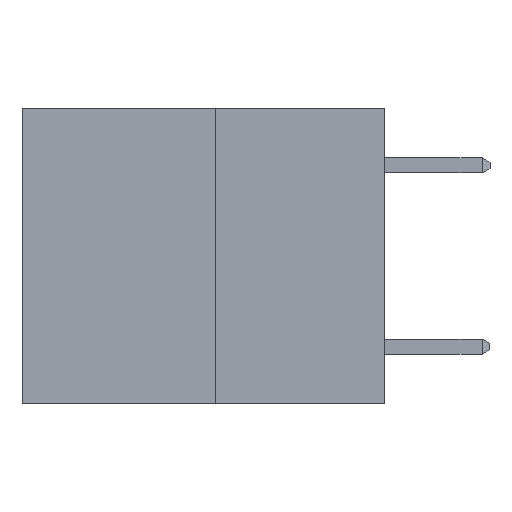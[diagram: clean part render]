
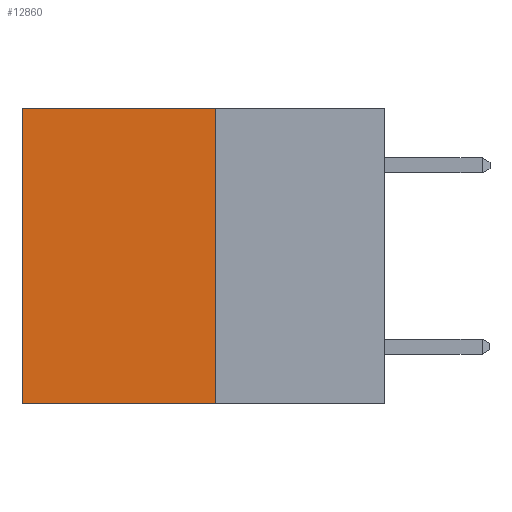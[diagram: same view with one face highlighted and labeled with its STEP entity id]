
A CAD part, left-side view. The second image highlights one B-rep face of the part: STEP entity #12860.
In plain terms, the highlighted planar face has unit normal (-1, 0, 0).
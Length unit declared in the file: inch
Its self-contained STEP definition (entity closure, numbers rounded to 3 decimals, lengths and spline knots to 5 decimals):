
#2913 = VECTOR ( 'NONE', #9610, 39.37008 ) ;
#2992 = DIRECTION ( 'NONE',  ( 1., 0., 0. ) ) ;
#3046 = PLANE ( 'NONE',  #13994 ) ;
#3381 = LINE ( 'NONE', #11117, #15127 ) ;
#3393 = VERTEX_POINT ( 'NONE', #4233 ) ;
#4233 = CARTESIAN_POINT ( 'NONE',  ( 0.3165, 0.6, 0. ) ) ;
#4280 = EDGE_CURVE ( 'NONE', #5433, #3393, #3381, .T. ) ;
#4576 = CARTESIAN_POINT ( 'NONE',  ( 0.3165, 0.28, -0.49 ) ) ;
#4793 = ORIENTED_EDGE ( 'NONE', *, *, #9479, .F. ) ;
#4972 = VERTEX_POINT ( 'NONE', #5380 ) ;
#5353 = VECTOR ( 'NONE', #8446, 39.37008 ) ;
#5380 = CARTESIAN_POINT ( 'NONE',  ( 0.3165, 0.28, -0.49 ) ) ;
#5433 = VERTEX_POINT ( 'NONE', #14545 ) ;
#6951 = CARTESIAN_POINT ( 'NONE',  ( 0.3165, 0.28, -0.49 ) ) ;
#7068 = DIRECTION ( 'NONE',  ( 0., 0., -1. ) ) ;
#8384 = CARTESIAN_POINT ( 'NONE',  ( 0.3165, 0.28, -0.49 ) ) ;
#8446 = DIRECTION ( 'NONE',  ( 0., 1., 0. ) ) ;
#9214 = ORIENTED_EDGE ( 'NONE', *, *, #10001, .F. ) ;
#9479 = EDGE_CURVE ( 'NONE', #5433, #4972, #9801, .T. ) ;
#9610 = DIRECTION ( 'NONE',  ( 0., 0., -1. ) ) ;
#9801 = LINE ( 'NONE', #4576, #2913 ) ;
#9836 = ORIENTED_EDGE ( 'NONE', *, *, #10253, .T. ) ;
#10001 = EDGE_CURVE ( 'NONE', #4972, #16556, #12008, .T. ) ;
#10173 = LINE ( 'NONE', #12818, #12632 ) ;
#10253 = EDGE_CURVE ( 'NONE', #3393, #16556, #10173, .T. ) ;
#11117 = CARTESIAN_POINT ( 'NONE',  ( 0.3165, 0.28, 0. ) ) ;
#12008 = LINE ( 'NONE', #6951, #5353 ) ;
#12233 = CARTESIAN_POINT ( 'NONE',  ( 0.3165, 0.6, -0.49 ) ) ;
#12632 = VECTOR ( 'NONE', #12861, 39.37008 ) ;
#12742 = FACE_OUTER_BOUND ( 'NONE', #14784, .T. ) ;
#12818 = CARTESIAN_POINT ( 'NONE',  ( 0.3165, 0.6, -0.49 ) ) ;
#12860 = ADVANCED_FACE ( 'NONE', ( #12742 ), #3046, .F. ) ;
#12861 = DIRECTION ( 'NONE',  ( 0., 0., -1. ) ) ;
#13994 = AXIS2_PLACEMENT_3D ( 'NONE', #8384, #2992, #7068 ) ;
#14545 = CARTESIAN_POINT ( 'NONE',  ( 0.3165, 0.28, 0. ) ) ;
#14784 = EDGE_LOOP ( 'NONE', ( #9836, #9214, #4793, #16172 ) ) ;
#15127 = VECTOR ( 'NONE', #15138, 39.37008 ) ;
#15138 = DIRECTION ( 'NONE',  ( 0., 1., 0. ) ) ;
#16172 = ORIENTED_EDGE ( 'NONE', *, *, #4280, .T. ) ;
#16556 = VERTEX_POINT ( 'NONE', #12233 ) ;
